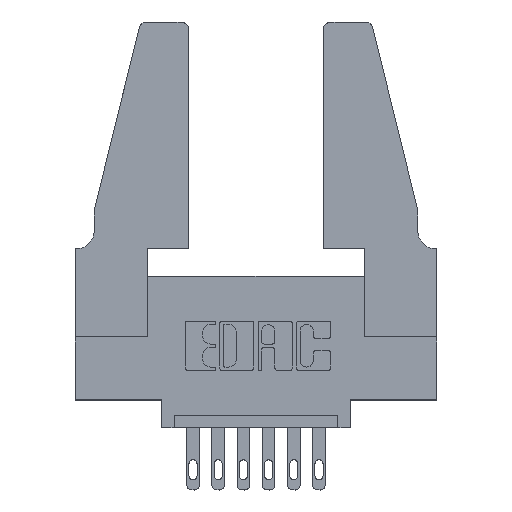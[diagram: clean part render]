
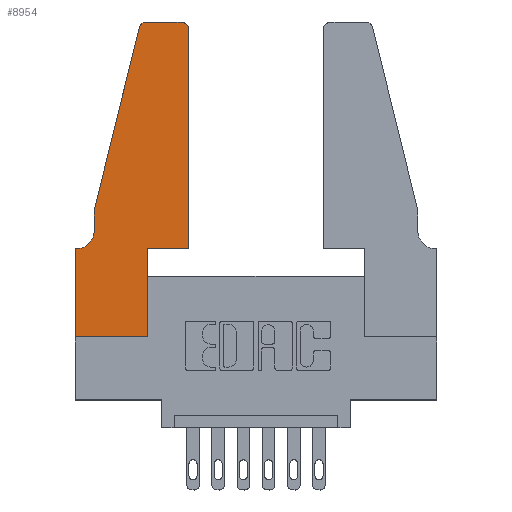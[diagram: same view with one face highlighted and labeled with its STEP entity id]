
A CAD part, top view. The second image highlights one B-rep face of the part: STEP entity #8954.
In plain terms, the highlighted planar face has unit normal (0, 0, 1).
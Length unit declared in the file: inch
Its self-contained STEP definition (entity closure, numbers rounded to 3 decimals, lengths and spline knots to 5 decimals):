
#205 = ORIENTED_EDGE ( 'NONE', *, *, #11519, .T. ) ;
#367 = DIRECTION ( 'NONE',  ( 0., 0., -1. ) ) ;
#389 = DIRECTION ( 'NONE',  ( 1., 0., 0. ) ) ;
#446 = CARTESIAN_POINT ( 'NONE',  ( 0., 0.35, 0.37 ) ) ;
#489 = DIRECTION ( 'NONE',  ( 0., -1., 0. ) ) ;
#538 = VERTEX_POINT ( 'NONE', #11016 ) ;
#795 = EDGE_CURVE ( 'NONE', #5228, #538, #3281, .T. ) ;
#915 = EDGE_CURVE ( 'NONE', #538, #2628, #6490, .T. ) ;
#1130 = ORIENTED_EDGE ( 'NONE', *, *, #2334, .T. ) ;
#1549 = CARTESIAN_POINT ( 'NONE',  ( 0.2865, 0.35, 0.37 ) ) ;
#1580 = ORIENTED_EDGE ( 'NONE', *, *, #5338, .T. ) ;
#1597 = ORIENTED_EDGE ( 'NONE', *, *, #4748, .T. ) ;
#1707 = DIRECTION ( 'NONE',  ( 1., 0., 0. ) ) ;
#1758 = VERTEX_POINT ( 'NONE', #2362 ) ;
#1779 = VERTEX_POINT ( 'NONE', #11425 ) ;
#1818 = CARTESIAN_POINT ( 'NONE',  ( 0.4505, 0.35, 0.37 ) ) ;
#1911 = ORIENTED_EDGE ( 'NONE', *, *, #4637, .T. ) ;
#2082 = LINE ( 'NONE', #10568, #10352 ) ;
#2185 = CIRCLE ( 'NONE', #3138, 0.03 ) ;
#2328 = DIRECTION ( 'NONE',  ( 0., 0., 1. ) ) ;
#2334 = EDGE_CURVE ( 'NONE', #7910, #10104, #3647, .T. ) ;
#2362 = CARTESIAN_POINT ( 'NONE',  ( 0.284, 1.25, 0.37 ) ) ;
#2616 = EDGE_LOOP ( 'NONE', ( #5835, #1597, #6479, #205, #7369, #11478, #1130, #1580, #1911, #8084, #8769, #10793 ) ) ;
#2628 = VERTEX_POINT ( 'NONE', #6579 ) ;
#2662 = DIRECTION ( 'NONE',  ( 1., 0., 0. ) ) ;
#2718 = CARTESIAN_POINT ( 'NONE',  ( 0.4505, 0.35, 0.37 ) ) ;
#2893 = AXIS2_PLACEMENT_3D ( 'NONE', #8350, #367, #5624 ) ;
#2979 = CARTESIAN_POINT ( 'NONE',  ( 0.4205, 1.22, 0.37 ) ) ;
#3024 = VECTOR ( 'NONE', #4007, 39.37008 ) ;
#3028 = DIRECTION ( 'NONE',  ( -1., 0., 0. ) ) ;
#3138 = AXIS2_PLACEMENT_3D ( 'NONE', #9287, #4064, #11133 ) ;
#3281 = LINE ( 'NONE', #1818, #10730 ) ;
#3430 = VERTEX_POINT ( 'NONE', #5986 ) ;
#3589 = CARTESIAN_POINT ( 'NONE',  ( 0.4505, 0.35, 0.37 ) ) ;
#3600 = LINE ( 'NONE', #1549, #3024 ) ;
#3647 = LINE ( 'NONE', #11281, #8969 ) ;
#3849 = EDGE_CURVE ( 'NONE', #11404, #5228, #8359, .T. ) ;
#4007 = DIRECTION ( 'NONE',  ( 0., 1., 0. ) ) ;
#4064 = DIRECTION ( 'NONE',  ( 0., 0., 1. ) ) ;
#4089 = VECTOR ( 'NONE', #4125, 39.37008 ) ;
#4125 = DIRECTION ( 'NONE',  ( -0.239, -0.971, 0. ) ) ;
#4197 = VECTOR ( 'NONE', #489, 39.37008 ) ;
#4232 = LINE ( 'NONE', #10555, #4089 ) ;
#4306 = VERTEX_POINT ( 'NONE', #11458 ) ;
#4349 = CIRCLE ( 'NONE', #2893, 0.07 ) ;
#4633 = CARTESIAN_POINT ( 'NONE',  ( 0.0055, 0.35, 0.37 ) ) ;
#4637 = EDGE_CURVE ( 'NONE', #1779, #11404, #3600, .T. ) ;
#4748 = EDGE_CURVE ( 'NONE', #1758, #4306, #2185, .T. ) ;
#4890 = DIRECTION ( 'NONE',  ( 1., 0., 0. ) ) ;
#4979 = VECTOR ( 'NONE', #1707, 39.37008 ) ;
#5067 = VERTEX_POINT ( 'NONE', #4633 ) ;
#5228 = VERTEX_POINT ( 'NONE', #2718 ) ;
#5338 = EDGE_CURVE ( 'NONE', #10104, #1779, #6793, .T. ) ;
#5624 = DIRECTION ( 'NONE',  ( -1., 0., 0. ) ) ;
#5777 = PLANE ( 'NONE',  #8284 ) ;
#5835 = ORIENTED_EDGE ( 'NONE', *, *, #11443, .T. ) ;
#5986 = CARTESIAN_POINT ( 'NONE',  ( 0.0755, 0.42, 0.37 ) ) ;
#6100 = EDGE_CURVE ( 'NONE', #4306, #9384, #4232, .T. ) ;
#6447 = CARTESIAN_POINT ( 'NONE',  ( 0.2865, 0.35, 0.37 ) ) ;
#6479 = ORIENTED_EDGE ( 'NONE', *, *, #6100, .T. ) ;
#6490 = CIRCLE ( 'NONE', #10719, 0.03 ) ;
#6579 = CARTESIAN_POINT ( 'NONE',  ( 0.4205, 1.25, 0.37 ) ) ;
#6760 = CARTESIAN_POINT ( 'NONE',  ( 0., 0.35, 0.37 ) ) ;
#6793 = LINE ( 'NONE', #8018, #10600 ) ;
#7155 = LINE ( 'NONE', #7683, #4197 ) ;
#7369 = ORIENTED_EDGE ( 'NONE', *, *, #11397, .T. ) ;
#7419 = VECTOR ( 'NONE', #3028, 39.37008 ) ;
#7683 = CARTESIAN_POINT ( 'NONE',  ( 0.0755, 0.5, 0.37 ) ) ;
#7910 = VERTEX_POINT ( 'NONE', #6760 ) ;
#7995 = LINE ( 'NONE', #11024, #7419 ) ;
#8018 = CARTESIAN_POINT ( 'NONE',  ( 0., 0., 0.37 ) ) ;
#8084 = ORIENTED_EDGE ( 'NONE', *, *, #3849, .T. ) ;
#8284 = AXIS2_PLACEMENT_3D ( 'NONE', #446, #2328, #4890 ) ;
#8350 = CARTESIAN_POINT ( 'NONE',  ( 0.0055, 0.42, 0.37 ) ) ;
#8359 = LINE ( 'NONE', #3589, #4979 ) ;
#8610 = DIRECTION ( 'NONE',  ( 0., -1., 0. ) ) ;
#8769 = ORIENTED_EDGE ( 'NONE', *, *, #795, .T. ) ;
#8783 = DIRECTION ( 'NONE',  ( -1., 0., 0. ) ) ;
#8954 = ADVANCED_FACE ( 'NONE', ( #11047 ), #5777, .T. ) ;
#8969 = VECTOR ( 'NONE', #8610, 39.37008 ) ;
#9001 = DIRECTION ( 'NONE',  ( 0., 1., 0. ) ) ;
#9287 = CARTESIAN_POINT ( 'NONE',  ( 0.284, 1.22, 0.37 ) ) ;
#9384 = VERTEX_POINT ( 'NONE', #9621 ) ;
#9555 = CARTESIAN_POINT ( 'NONE',  ( 0., 0., 0.37 ) ) ;
#9621 = CARTESIAN_POINT ( 'NONE',  ( 0.0755, 0.5, 0.37 ) ) ;
#9974 = EDGE_CURVE ( 'NONE', #5067, #7910, #2082, .T. ) ;
#10104 = VERTEX_POINT ( 'NONE', #9555 ) ;
#10352 = VECTOR ( 'NONE', #8783, 39.37008 ) ;
#10555 = CARTESIAN_POINT ( 'NONE',  ( 0.0755, 0.5, 0.37 ) ) ;
#10568 = CARTESIAN_POINT ( 'NONE',  ( 0.0755, 0.35, 0.37 ) ) ;
#10600 = VECTOR ( 'NONE', #2662, 39.37008 ) ;
#10719 = AXIS2_PLACEMENT_3D ( 'NONE', #2979, #11089, #389 ) ;
#10730 = VECTOR ( 'NONE', #9001, 39.37008 ) ;
#10793 = ORIENTED_EDGE ( 'NONE', *, *, #915, .T. ) ;
#11016 = CARTESIAN_POINT ( 'NONE',  ( 0.4505, 1.22, 0.37 ) ) ;
#11024 = CARTESIAN_POINT ( 'NONE',  ( 0.2605, 1.25, 0.37 ) ) ;
#11047 = FACE_OUTER_BOUND ( 'NONE', #2616, .T. ) ;
#11089 = DIRECTION ( 'NONE',  ( 0., 0., 1. ) ) ;
#11133 = DIRECTION ( 'NONE',  ( 1., 0., 0. ) ) ;
#11281 = CARTESIAN_POINT ( 'NONE',  ( 0., 0., 0.37 ) ) ;
#11397 = EDGE_CURVE ( 'NONE', #3430, #5067, #4349, .T. ) ;
#11404 = VERTEX_POINT ( 'NONE', #6447 ) ;
#11425 = CARTESIAN_POINT ( 'NONE',  ( 0.2865, 0., 0.37 ) ) ;
#11443 = EDGE_CURVE ( 'NONE', #2628, #1758, #7995, .T. ) ;
#11458 = CARTESIAN_POINT ( 'NONE',  ( 0.25487, 1.22718, 0.37 ) ) ;
#11478 = ORIENTED_EDGE ( 'NONE', *, *, #9974, .T. ) ;
#11519 = EDGE_CURVE ( 'NONE', #9384, #3430, #7155, .T. ) ;
